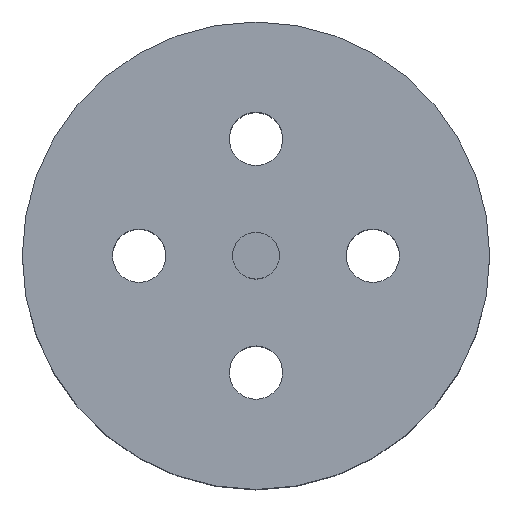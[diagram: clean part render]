
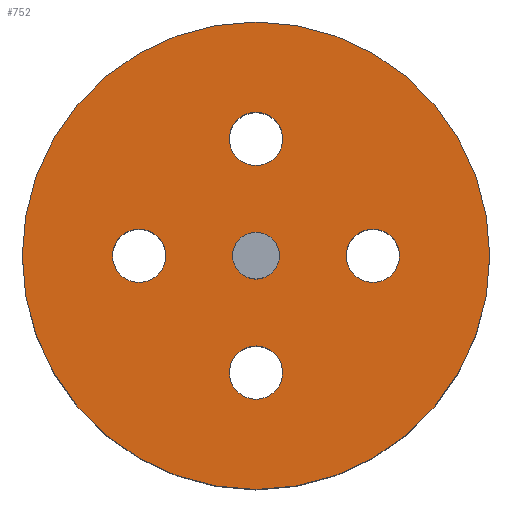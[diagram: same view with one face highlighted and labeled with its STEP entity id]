
A CAD part, top view. The second image highlights one B-rep face of the part: STEP entity #752.
In plain terms, the highlighted planar face has unit normal (0, 0, 1).
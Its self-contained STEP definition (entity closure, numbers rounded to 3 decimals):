
#166 = CARTESIAN_POINT ( 'NONE',  ( 0., 12.5, 30. ) ) ;
#167 = DIRECTION ( 'NONE',  ( 0., 0., -1. ) ) ;
#168 = DIRECTION ( 'NONE',  ( -1., 0., 0. ) ) ;
#177 = CARTESIAN_POINT ( 'NONE',  ( -12.5, 0., 30. ) ) ;
#178 = DIRECTION ( 'NONE',  ( 0., 0., 1. ) ) ;
#179 = DIRECTION ( 'NONE',  ( 1., 0., 0. ) ) ;
#187 = CARTESIAN_POINT ( 'NONE',  ( 0., -12.5, 30. ) ) ;
#188 = DIRECTION ( 'NONE',  ( 0., 0., 1. ) ) ;
#189 = DIRECTION ( 'NONE',  ( 1., 0., 0. ) ) ;
#197 = CARTESIAN_POINT ( 'NONE',  ( 12.5, 0., 30. ) ) ;
#198 = DIRECTION ( 'NONE',  ( 0., 0., 1. ) ) ;
#199 = DIRECTION ( 'NONE',  ( 1., 0., 0. ) ) ;
#210 = CARTESIAN_POINT ( 'NONE',  ( 0., 0., 30. ) ) ;
#211 = DIRECTION ( 'NONE',  ( 0., 0., 1. ) ) ;
#212 = DIRECTION ( 'NONE',  ( 1., 0., 0. ) ) ;
#216 = CARTESIAN_POINT ( 'NONE',  ( 0., 0., 30. ) ) ;
#217 = DIRECTION ( 'NONE',  ( 0., 0., 1. ) ) ;
#218 = DIRECTION ( 'NONE',  ( 1., 0., 0. ) ) ;
#380 = FACE_BOUND ( 'NONE', #1339, .T. ) ;
#381 = FACE_BOUND ( 'NONE', #1328, .T. ) ;
#382 = FACE_OUTER_BOUND ( 'NONE', #1342, .T. ) ;
#383 = FACE_BOUND ( 'NONE', #1335, .T. ) ;
#384 = FACE_BOUND ( 'NONE', #1337, .T. ) ;
#385 = FACE_BOUND ( 'NONE', #1336, .T. ) ;
#458 = CIRCLE ( 'NONE', #664, 2.85 ) ;
#461 = CIRCLE ( 'NONE', #666, 2.85 ) ;
#470 = CIRCLE ( 'NONE', #668, 2.85 ) ;
#472 = CIRCLE ( 'NONE', #673, 2.85 ) ;
#484 = CIRCLE ( 'NONE', #676, 2.5 ) ;
#485 = CIRCLE ( 'NONE', #677, 25. ) ;
#556 = CIRCLE ( 'NONE', #697, 2.85 ) ;
#557 = CIRCLE ( 'NONE', #698, 2.85 ) ;
#558 = CIRCLE ( 'NONE', #699, 2.85 ) ;
#559 = CIRCLE ( 'NONE', #700, 2.85 ) ;
#560 = CIRCLE ( 'NONE', #701, 25. ) ;
#561 = CIRCLE ( 'NONE', #702, 2.5 ) ;
#625 = AXIS2_PLACEMENT_3D ( 'NONE', #920, #912, #922 ) ;
#664 = AXIS2_PLACEMENT_3D ( 'NONE', #166, #167, #168 ) ;
#666 = AXIS2_PLACEMENT_3D ( 'NONE', #177, #178, #179 ) ;
#668 = AXIS2_PLACEMENT_3D ( 'NONE', #187, #188, #189 ) ;
#673 = AXIS2_PLACEMENT_3D ( 'NONE', #197, #198, #199 ) ;
#676 = AXIS2_PLACEMENT_3D ( 'NONE', #210, #211, #212 ) ;
#677 = AXIS2_PLACEMENT_3D ( 'NONE', #216, #217, #218 ) ;
#697 = AXIS2_PLACEMENT_3D ( 'NONE', #1463, #1464, #1465 ) ;
#698 = AXIS2_PLACEMENT_3D ( 'NONE', #1466, #1467, #1468 ) ;
#699 = AXIS2_PLACEMENT_3D ( 'NONE', #1469, #1470, #1471 ) ;
#700 = AXIS2_PLACEMENT_3D ( 'NONE', #1472, #1473, #1474 ) ;
#701 = AXIS2_PLACEMENT_3D ( 'NONE', #1475, #1476, #1477 ) ;
#702 = AXIS2_PLACEMENT_3D ( 'NONE', #1478, #1479, #1480 ) ;
#752 = ADVANCED_FACE ( 'NONE', ( #380, #384, #381, #383, #382, #385 ), #919, .T. ) ;
#912 = DIRECTION ( 'NONE',  ( 0., 0., 1. ) ) ;
#919 = PLANE ( 'NONE',  #625 ) ;
#920 = CARTESIAN_POINT ( 'NONE',  ( 0., 0., 30. ) ) ;
#922 = DIRECTION ( 'NONE',  ( 1., 0., 0. ) ) ;
#1012 = EDGE_CURVE ( 'NONE', #1141, #1186, #458, .T. ) ;
#1016 = EDGE_CURVE ( 'NONE', #1144, #1145, #461, .T. ) ;
#1020 = EDGE_CURVE ( 'NONE', #1148, #1149, #470, .T. ) ;
#1024 = EDGE_CURVE ( 'NONE', #1152, #1153, #472, .T. ) ;
#1030 = EDGE_CURVE ( 'NONE', #1164, #1171, #484, .T. ) ;
#1032 = EDGE_CURVE ( 'NONE', #1162, #1163, #485, .T. ) ;
#1076 = EDGE_CURVE ( 'NONE', #1186, #1141, #556, .T. ) ;
#1077 = EDGE_CURVE ( 'NONE', #1145, #1144, #557, .T. ) ;
#1078 = EDGE_CURVE ( 'NONE', #1149, #1148, #558, .T. ) ;
#1079 = EDGE_CURVE ( 'NONE', #1153, #1152, #559, .T. ) ;
#1080 = EDGE_CURVE ( 'NONE', #1163, #1162, #560, .T. ) ;
#1081 = EDGE_CURVE ( 'NONE', #1171, #1164, #561, .T. ) ;
#1092 = ORIENTED_EDGE ( 'NONE', *, *, #1076, .T. ) ;
#1093 = ORIENTED_EDGE ( 'NONE', *, *, #1012, .T. ) ;
#1094 = ORIENTED_EDGE ( 'NONE', *, *, #1016, .F. ) ;
#1095 = ORIENTED_EDGE ( 'NONE', *, *, #1077, .F. ) ;
#1096 = ORIENTED_EDGE ( 'NONE', *, *, #1020, .F. ) ;
#1097 = ORIENTED_EDGE ( 'NONE', *, *, #1078, .F. ) ;
#1098 = ORIENTED_EDGE ( 'NONE', *, *, #1024, .F. ) ;
#1099 = ORIENTED_EDGE ( 'NONE', *, *, #1079, .F. ) ;
#1100 = ORIENTED_EDGE ( 'NONE', *, *, #1080, .T. ) ;
#1101 = ORIENTED_EDGE ( 'NONE', *, *, #1032, .T. ) ;
#1102 = ORIENTED_EDGE ( 'NONE', *, *, #1081, .F. ) ;
#1103 = ORIENTED_EDGE ( 'NONE', *, *, #1030, .F. ) ;
#1141 = VERTEX_POINT ( 'NONE', #1499 ) ;
#1144 = VERTEX_POINT ( 'NONE', #1493 ) ;
#1145 = VERTEX_POINT ( 'NONE', #1501 ) ;
#1148 = VERTEX_POINT ( 'NONE', #1504 ) ;
#1149 = VERTEX_POINT ( 'NONE', #1505 ) ;
#1152 = VERTEX_POINT ( 'NONE', #1508 ) ;
#1153 = VERTEX_POINT ( 'NONE', #1509 ) ;
#1162 = VERTEX_POINT ( 'NONE', #1518 ) ;
#1163 = VERTEX_POINT ( 'NONE', #1519 ) ;
#1164 = VERTEX_POINT ( 'NONE', #1520 ) ;
#1171 = VERTEX_POINT ( 'NONE', #1527 ) ;
#1186 = VERTEX_POINT ( 'NONE', #1542 ) ;
#1328 = EDGE_LOOP ( 'NONE', ( #1096, #1097 ) ) ;
#1335 = EDGE_LOOP ( 'NONE', ( #1098, #1099 ) ) ;
#1336 = EDGE_LOOP ( 'NONE', ( #1102, #1103 ) ) ;
#1337 = EDGE_LOOP ( 'NONE', ( #1094, #1095 ) ) ;
#1339 = EDGE_LOOP ( 'NONE', ( #1092, #1093 ) ) ;
#1342 = EDGE_LOOP ( 'NONE', ( #1100, #1101 ) ) ;
#1463 = CARTESIAN_POINT ( 'NONE',  ( 0., 12.5, 30. ) ) ;
#1464 = DIRECTION ( 'NONE',  ( 0., 0., -1. ) ) ;
#1465 = DIRECTION ( 'NONE',  ( -1., 0., 0. ) ) ;
#1466 = CARTESIAN_POINT ( 'NONE',  ( -12.5, 0., 30. ) ) ;
#1467 = DIRECTION ( 'NONE',  ( 0., 0., 1. ) ) ;
#1468 = DIRECTION ( 'NONE',  ( 1., 0., 0. ) ) ;
#1469 = CARTESIAN_POINT ( 'NONE',  ( 0., -12.5, 30. ) ) ;
#1470 = DIRECTION ( 'NONE',  ( 0., 0., 1. ) ) ;
#1471 = DIRECTION ( 'NONE',  ( 1., 0., 0. ) ) ;
#1472 = CARTESIAN_POINT ( 'NONE',  ( 12.5, 0., 30. ) ) ;
#1473 = DIRECTION ( 'NONE',  ( 0., 0., 1. ) ) ;
#1474 = DIRECTION ( 'NONE',  ( 1., 0., 0. ) ) ;
#1475 = CARTESIAN_POINT ( 'NONE',  ( 0., 0., 30. ) ) ;
#1476 = DIRECTION ( 'NONE',  ( 0., 0., 1. ) ) ;
#1477 = DIRECTION ( 'NONE',  ( 1., 0., 0. ) ) ;
#1478 = CARTESIAN_POINT ( 'NONE',  ( 0., 0., 30. ) ) ;
#1479 = DIRECTION ( 'NONE',  ( 0., 0., 1. ) ) ;
#1480 = DIRECTION ( 'NONE',  ( 1., 0., 0. ) ) ;
#1493 = CARTESIAN_POINT ( 'NONE',  ( -15.35, 0., 30. ) ) ;
#1499 = CARTESIAN_POINT ( 'NONE',  ( 2.85, 12.5, 30. ) ) ;
#1501 = CARTESIAN_POINT ( 'NONE',  ( -9.65, 0., 30. ) ) ;
#1504 = CARTESIAN_POINT ( 'NONE',  ( -2.85, -12.5, 30. ) ) ;
#1505 = CARTESIAN_POINT ( 'NONE',  ( 2.85, -12.5, 30. ) ) ;
#1508 = CARTESIAN_POINT ( 'NONE',  ( 9.65, 0., 30. ) ) ;
#1509 = CARTESIAN_POINT ( 'NONE',  ( 15.35, 0., 30. ) ) ;
#1518 = CARTESIAN_POINT ( 'NONE',  ( 25., 0., 30. ) ) ;
#1519 = CARTESIAN_POINT ( 'NONE',  ( -25., 0., 30. ) ) ;
#1520 = CARTESIAN_POINT ( 'NONE',  ( 2.5, 0., 30. ) ) ;
#1527 = CARTESIAN_POINT ( 'NONE',  ( -2.5, 0., 30. ) ) ;
#1542 = CARTESIAN_POINT ( 'NONE',  ( -2.85, 12.5, 30. ) ) ;
